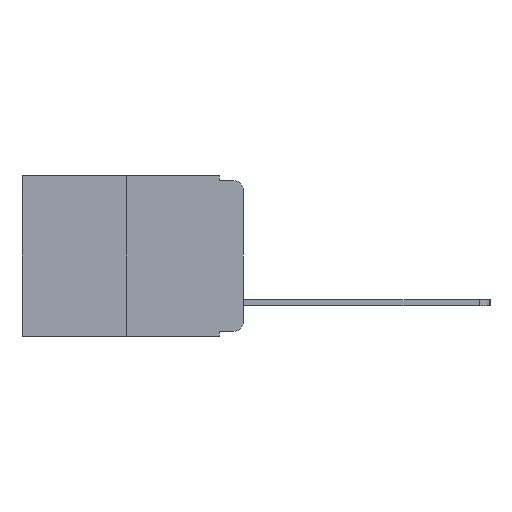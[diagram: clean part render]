
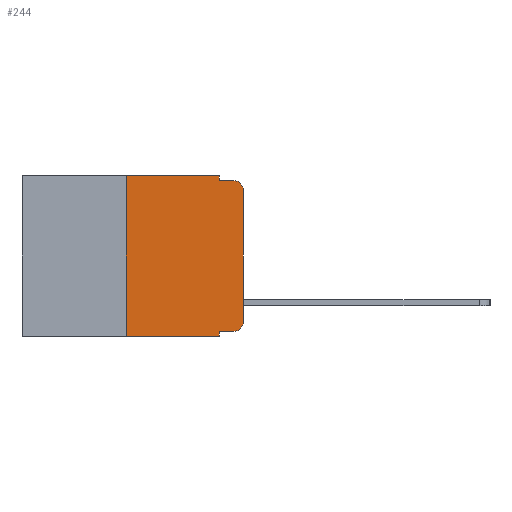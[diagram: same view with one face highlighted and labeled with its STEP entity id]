
A CAD part, left-side view. The second image highlights one B-rep face of the part: STEP entity #244.
In plain terms, the highlighted planar face has unit normal (-1, 0, 0).
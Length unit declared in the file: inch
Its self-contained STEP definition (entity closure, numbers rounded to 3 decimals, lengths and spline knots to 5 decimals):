
#244 = ADVANCED_FACE ( 'NONE', ( #5599 ), #5231, .F. ) ;
#251 = ORIENTED_EDGE ( 'NONE', *, *, #10440, .T. ) ;
#253 = EDGE_CURVE ( 'NONE', #10215, #5507, #9746, .T. ) ;
#462 = DIRECTION ( 'NONE',  ( 0., 0., 1. ) ) ;
#521 = DIRECTION ( 'NONE',  ( 0., 0., -1. ) ) ;
#633 = ORIENTED_EDGE ( 'NONE', *, *, #877, .F. ) ;
#804 = CARTESIAN_POINT ( 'NONE',  ( 0., 0.051, -0.333 ) ) ;
#877 = EDGE_CURVE ( 'NONE', #5900, #4204, #4219, .T. ) ;
#883 = ORIENTED_EDGE ( 'NONE', *, *, #253, .F. ) ;
#986 = EDGE_LOOP ( 'NONE', ( #1497, #1121, #2255, #633, #2582, #883, #1859, #4442, #251, #8277 ) ) ;
#1045 = LINE ( 'NONE', #6131, #10041 ) ;
#1121 = ORIENTED_EDGE ( 'NONE', *, *, #2799, .T. ) ;
#1460 = VECTOR ( 'NONE', #521, 39.37008 ) ;
#1497 = ORIENTED_EDGE ( 'NONE', *, *, #3410, .T. ) ;
#1520 = EDGE_CURVE ( 'NONE', #4204, #3070, #9860, .T. ) ;
#1523 = CARTESIAN_POINT ( 'NONE',  ( 0., 0.25, 0. ) ) ;
#1571 = VECTOR ( 'NONE', #10906, 39.37008 ) ;
#1747 = CARTESIAN_POINT ( 'NONE',  ( 0., 0.051, -0.01 ) ) ;
#1859 = ORIENTED_EDGE ( 'NONE', *, *, #6130, .T. ) ;
#2183 = CARTESIAN_POINT ( 'NONE',  ( 0., 0.051, 0. ) ) ;
#2200 = CIRCLE ( 'NONE', #10608, 0.02 ) ;
#2255 = ORIENTED_EDGE ( 'NONE', *, *, #1520, .F. ) ;
#2582 = ORIENTED_EDGE ( 'NONE', *, *, #5816, .F. ) ;
#2799 = EDGE_CURVE ( 'NONE', #4083, #3070, #8608, .T. ) ;
#3070 = VERTEX_POINT ( 'NONE', #7222 ) ;
#3410 = EDGE_CURVE ( 'NONE', #9364, #4083, #11261, .T. ) ;
#3588 = AXIS2_PLACEMENT_3D ( 'NONE', #10758, #7369, #5608 ) ;
#3780 = LINE ( 'NONE', #804, #8248 ) ;
#4043 = VECTOR ( 'NONE', #462, 39.37008 ) ;
#4069 = CARTESIAN_POINT ( 'NONE',  ( 0., 0.02, -0.313 ) ) ;
#4083 = VERTEX_POINT ( 'NONE', #4788 ) ;
#4204 = VERTEX_POINT ( 'NONE', #9828 ) ;
#4219 = LINE ( 'NONE', #9003, #1460 ) ;
#4282 = VERTEX_POINT ( 'NONE', #10160 ) ;
#4442 = ORIENTED_EDGE ( 'NONE', *, *, #10987, .F. ) ;
#4476 = CARTESIAN_POINT ( 'NONE',  ( 0., 0.02, -0.03 ) ) ;
#4505 = AXIS2_PLACEMENT_3D ( 'NONE', #4476, #11154, #7262 ) ;
#4654 = DIRECTION ( 'NONE',  ( 0., 0., 1. ) ) ;
#4757 = CARTESIAN_POINT ( 'NONE',  ( 0., 0.473, 0. ) ) ;
#4774 = VERTEX_POINT ( 'NONE', #10340 ) ;
#4788 = CARTESIAN_POINT ( 'NONE',  ( 0., 0., -0.03 ) ) ;
#4948 = DIRECTION ( 'NONE',  ( 0., 0., -1. ) ) ;
#5032 = CARTESIAN_POINT ( 'NONE',  ( 0., 0.051, 0. ) ) ;
#5081 = CARTESIAN_POINT ( 'NONE',  ( 0., 0.25, -0.343 ) ) ;
#5231 = PLANE ( 'NONE',  #3588 ) ;
#5391 = CARTESIAN_POINT ( 'NONE',  ( 0., 0.02, -0.333 ) ) ;
#5472 = CARTESIAN_POINT ( 'NONE',  ( 0., 0., 0. ) ) ;
#5507 = VERTEX_POINT ( 'NONE', #7292 ) ;
#5599 = FACE_OUTER_BOUND ( 'NONE', #986, .T. ) ;
#5608 = DIRECTION ( 'NONE',  ( 0., 0., -1. ) ) ;
#5816 = EDGE_CURVE ( 'NONE', #5507, #5900, #10055, .T. ) ;
#5897 = VECTOR ( 'NONE', #8239, 39.37008 ) ;
#5900 = VERTEX_POINT ( 'NONE', #2183 ) ;
#6130 = EDGE_CURVE ( 'NONE', #10215, #4774, #1045, .T. ) ;
#6131 = CARTESIAN_POINT ( 'NONE',  ( 0., 0.473, -0.343 ) ) ;
#6714 = CARTESIAN_POINT ( 'NONE',  ( 0., 0., -0.313 ) ) ;
#6794 = VERTEX_POINT ( 'NONE', #5391 ) ;
#7057 = DIRECTION ( 'NONE',  ( 0., -1., 0. ) ) ;
#7222 = CARTESIAN_POINT ( 'NONE',  ( 0., 0.02, -0.01 ) ) ;
#7262 = DIRECTION ( 'NONE',  ( 0., 0., -1. ) ) ;
#7292 = CARTESIAN_POINT ( 'NONE',  ( 0., 0.25, 0. ) ) ;
#7369 = DIRECTION ( 'NONE',  ( 1., 0., 0. ) ) ;
#7779 = VECTOR ( 'NONE', #8634, 39.37008 ) ;
#8226 = DIRECTION ( 'NONE',  ( 0., -1., 0. ) ) ;
#8239 = DIRECTION ( 'NONE',  ( 0., -1., 0. ) ) ;
#8248 = VECTOR ( 'NONE', #7057, 39.37008 ) ;
#8277 = ORIENTED_EDGE ( 'NONE', *, *, #9284, .T. ) ;
#8608 = CIRCLE ( 'NONE', #4505, 0.02 ) ;
#8634 = DIRECTION ( 'NONE',  ( 0., -1., 0. ) ) ;
#9003 = CARTESIAN_POINT ( 'NONE',  ( 0., 0.051, 0. ) ) ;
#9284 = EDGE_CURVE ( 'NONE', #6794, #9364, #2200, .T. ) ;
#9364 = VERTEX_POINT ( 'NONE', #6714 ) ;
#9475 = VECTOR ( 'NONE', #4654, 39.37008 ) ;
#9746 = LINE ( 'NONE', #1523, #9475 ) ;
#9828 = CARTESIAN_POINT ( 'NONE',  ( 0., 0.051, -0.01 ) ) ;
#9860 = LINE ( 'NONE', #1747, #7779 ) ;
#9962 = DIRECTION ( 'NONE',  ( -1., 0., 0. ) ) ;
#10041 = VECTOR ( 'NONE', #8226, 39.37008 ) ;
#10055 = LINE ( 'NONE', #4757, #5897 ) ;
#10160 = CARTESIAN_POINT ( 'NONE',  ( 0., 0.051, -0.333 ) ) ;
#10215 = VERTEX_POINT ( 'NONE', #5081 ) ;
#10239 = LINE ( 'NONE', #5032, #1571 ) ;
#10340 = CARTESIAN_POINT ( 'NONE',  ( 0., 0.051, -0.343 ) ) ;
#10440 = EDGE_CURVE ( 'NONE', #4282, #6794, #3780, .T. ) ;
#10608 = AXIS2_PLACEMENT_3D ( 'NONE', #4069, #9962, #4948 ) ;
#10758 = CARTESIAN_POINT ( 'NONE',  ( 0., 0.473, 0. ) ) ;
#10906 = DIRECTION ( 'NONE',  ( 0., 0., -1. ) ) ;
#10987 = EDGE_CURVE ( 'NONE', #4282, #4774, #10239, .T. ) ;
#11154 = DIRECTION ( 'NONE',  ( -1., 0., 0. ) ) ;
#11261 = LINE ( 'NONE', #5472, #4043 ) ;
